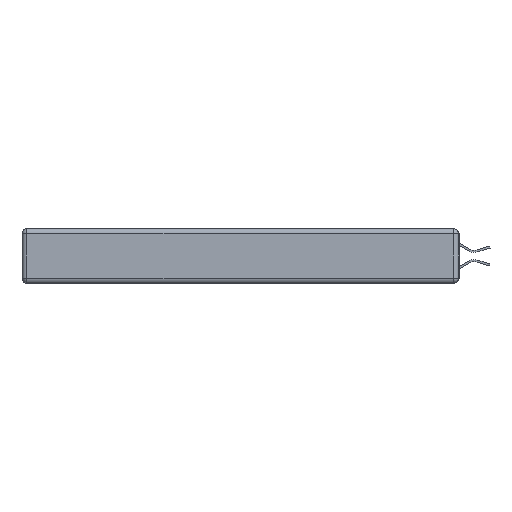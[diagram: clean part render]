
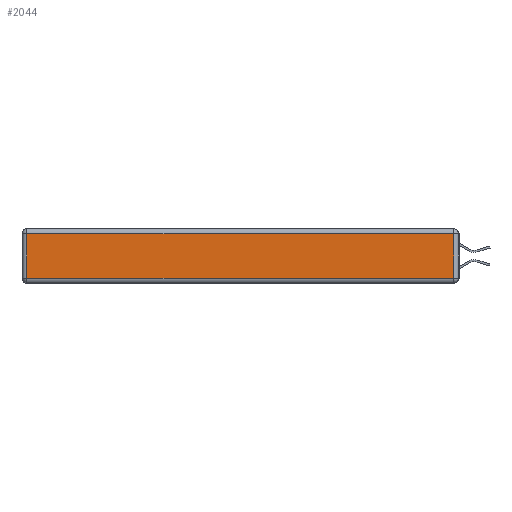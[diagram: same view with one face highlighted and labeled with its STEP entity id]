
A CAD part, left-side view. The second image highlights one B-rep face of the part: STEP entity #2044.
In plain terms, the highlighted planar face has unit normal (-1, 0, 0).
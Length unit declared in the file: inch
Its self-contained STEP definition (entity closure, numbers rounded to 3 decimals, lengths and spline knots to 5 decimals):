
#85 = CARTESIAN_POINT ( 'NONE',  ( 0., 0., -0.313 ) ) ;
#427 = ORIENTED_EDGE ( 'NONE', *, *, #9368, .T. ) ;
#548 = VECTOR ( 'NONE', #10732, 39.37008 ) ;
#706 = EDGE_LOOP ( 'NONE', ( #3909, #10532, #11115, #427 ) ) ;
#969 = CARTESIAN_POINT ( 'NONE',  ( 0., 0.03, -0.343 ) ) ;
#1159 = VECTOR ( 'NONE', #9055, 39.37008 ) ;
#1680 = DIRECTION ( 'NONE',  ( 0., 0., -1. ) ) ;
#1912 = VECTOR ( 'NONE', #4928, 39.37008 ) ;
#2044 = ADVANCED_FACE ( 'NONE', ( #3921 ), #12971, .T. ) ;
#3640 = VERTEX_POINT ( 'NONE', #5563 ) ;
#3909 = ORIENTED_EDGE ( 'NONE', *, *, #15242, .T. ) ;
#3921 = FACE_OUTER_BOUND ( 'NONE', #706, .T. ) ;
#4443 = CARTESIAN_POINT ( 'NONE',  ( 0., 2.72, -0.343 ) ) ;
#4454 = DIRECTION ( 'NONE',  ( 0., 0., 1. ) ) ;
#4739 = CARTESIAN_POINT ( 'NONE',  ( 0., 0.03, -0.313 ) ) ;
#4928 = DIRECTION ( 'NONE',  ( 0., -1., 0. ) ) ;
#5563 = CARTESIAN_POINT ( 'NONE',  ( 0., 2.72, -0.313 ) ) ;
#5575 = AXIS2_PLACEMENT_3D ( 'NONE', #15431, #10271, #4454 ) ;
#5837 = VERTEX_POINT ( 'NONE', #15398 ) ;
#6113 = LINE ( 'NONE', #85, #1912 ) ;
#7737 = CARTESIAN_POINT ( 'NONE',  ( 0., 0.03, -0.03 ) ) ;
#7919 = LINE ( 'NONE', #10405, #1159 ) ;
#8297 = VERTEX_POINT ( 'NONE', #7737 ) ;
#9055 = DIRECTION ( 'NONE',  ( 0., 1., 0. ) ) ;
#9368 = EDGE_CURVE ( 'NONE', #5837, #3640, #12714, .T. ) ;
#10271 = DIRECTION ( 'NONE',  ( -1., 0., 0. ) ) ;
#10405 = CARTESIAN_POINT ( 'NONE',  ( 0., 2.75, -0.03 ) ) ;
#10532 = ORIENTED_EDGE ( 'NONE', *, *, #12117, .T. ) ;
#10552 = EDGE_CURVE ( 'NONE', #8297, #5837, #7919, .T. ) ;
#10732 = DIRECTION ( 'NONE',  ( 0., 0., 1. ) ) ;
#11115 = ORIENTED_EDGE ( 'NONE', *, *, #10552, .T. ) ;
#12117 = EDGE_CURVE ( 'NONE', #13756, #8297, #12962, .T. ) ;
#12714 = LINE ( 'NONE', #4443, #14313 ) ;
#12962 = LINE ( 'NONE', #969, #548 ) ;
#12971 = PLANE ( 'NONE',  #5575 ) ;
#13756 = VERTEX_POINT ( 'NONE', #4739 ) ;
#14313 = VECTOR ( 'NONE', #1680, 39.37008 ) ;
#15242 = EDGE_CURVE ( 'NONE', #3640, #13756, #6113, .T. ) ;
#15398 = CARTESIAN_POINT ( 'NONE',  ( 0., 2.72, -0.03 ) ) ;
#15431 = CARTESIAN_POINT ( 'NONE',  ( 0., 0., -0.343 ) ) ;
